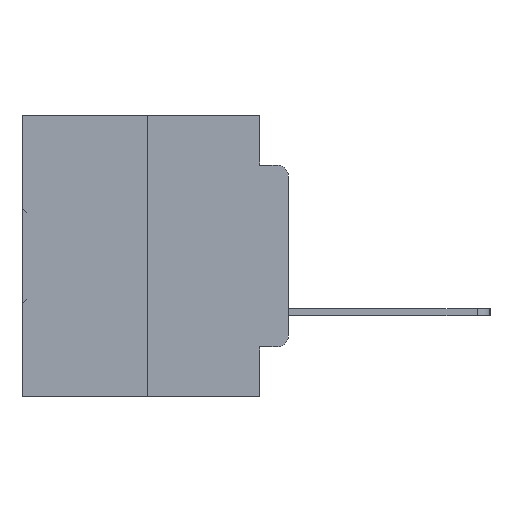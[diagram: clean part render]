
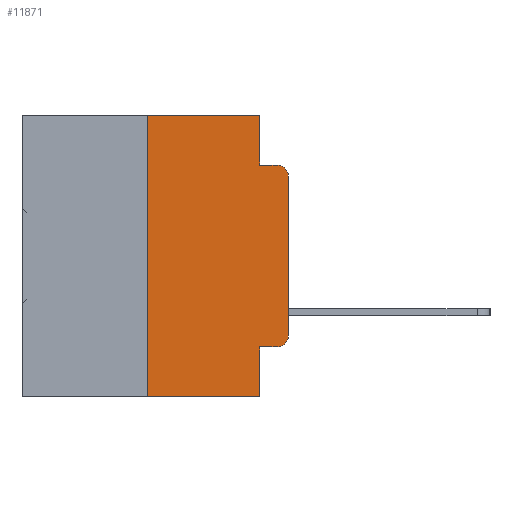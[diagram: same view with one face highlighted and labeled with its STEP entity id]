
A CAD part, left-side view. The second image highlights one B-rep face of the part: STEP entity #11871.
In plain terms, the highlighted planar face has unit normal (-1, 0, 0).
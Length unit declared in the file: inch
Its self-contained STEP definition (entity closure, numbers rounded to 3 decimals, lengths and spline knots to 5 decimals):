
#199 = DIRECTION ( 'NONE',  ( 0., 0., 1. ) ) ;
#475 = VERTEX_POINT ( 'NONE', #21425 ) ;
#478 = EDGE_CURVE ( 'NONE', #475, #26429, #2894, .T. ) ;
#1333 = LINE ( 'NONE', #27882, #20837 ) ;
#1368 = VERTEX_POINT ( 'NONE', #2451 ) ;
#2006 = CARTESIAN_POINT ( 'NONE',  ( 0., 0.051, -0.0885 ) ) ;
#2022 = LINE ( 'NONE', #18140, #21495 ) ;
#2107 = EDGE_CURVE ( 'NONE', #475, #4873, #27811, .T. ) ;
#2392 = CARTESIAN_POINT ( 'NONE',  ( 0., 0.051, 0. ) ) ;
#2451 = CARTESIAN_POINT ( 'NONE',  ( 0., 0., -0.3915 ) ) ;
#2533 = DIRECTION ( 'NONE',  ( 0., -1., 0. ) ) ;
#2737 = CARTESIAN_POINT ( 'NONE',  ( 0., 0.02, -0.4115 ) ) ;
#2894 = LINE ( 'NONE', #4148, #10009 ) ;
#4148 = CARTESIAN_POINT ( 'NONE',  ( 0., 0.25, 0. ) ) ;
#4685 = CARTESIAN_POINT ( 'NONE',  ( 0., 0.25, 0. ) ) ;
#4873 = VERTEX_POINT ( 'NONE', #21176 ) ;
#5117 = CARTESIAN_POINT ( 'NONE',  ( 0., 0., -0.1085 ) ) ;
#5927 = CARTESIAN_POINT ( 'NONE',  ( 0., 0.051, -0.4115 ) ) ;
#6429 = VERTEX_POINT ( 'NONE', #11936 ) ;
#6460 = ORIENTED_EDGE ( 'NONE', *, *, #12528, .T. ) ;
#6681 = VECTOR ( 'NONE', #19303, 39.37008 ) ;
#7149 = EDGE_LOOP ( 'NONE', ( #16428, #6460, #15190, #33262, #27308, #22845, #9764, #24481, #25291, #30917 ) ) ;
#7159 = EDGE_CURVE ( 'NONE', #1368, #19403, #1333, .T. ) ;
#8098 = CIRCLE ( 'NONE', #9084, 0.02 ) ;
#8668 = DIRECTION ( 'NONE',  ( 0., -1., 0. ) ) ;
#8931 = CARTESIAN_POINT ( 'NONE',  ( 0., 0.473, 0. ) ) ;
#9084 = AXIS2_PLACEMENT_3D ( 'NONE', #27501, #11947, #30055 ) ;
#9201 = CIRCLE ( 'NONE', #13900, 0.02 ) ;
#9411 = FACE_OUTER_BOUND ( 'NONE', #7149, .T. ) ;
#9418 = VERTEX_POINT ( 'NONE', #5927 ) ;
#9764 = ORIENTED_EDGE ( 'NONE', *, *, #2107, .T. ) ;
#10009 = VECTOR ( 'NONE', #199, 39.37008 ) ;
#10097 = DIRECTION ( 'NONE',  ( 0., -1., 0. ) ) ;
#11410 = VECTOR ( 'NONE', #10097, 39.37008 ) ;
#11652 = DIRECTION ( 'NONE',  ( 0., 0., -1. ) ) ;
#11871 = ADVANCED_FACE ( 'NONE', ( #9411 ), #22041, .F. ) ;
#11936 = CARTESIAN_POINT ( 'NONE',  ( 0., 0.02, -0.0885 ) ) ;
#11947 = DIRECTION ( 'NONE',  ( -1., 0., 0. ) ) ;
#12125 = VERTEX_POINT ( 'NONE', #2006 ) ;
#12528 = EDGE_CURVE ( 'NONE', #19403, #6429, #8098, .T. ) ;
#13048 = DIRECTION ( 'NONE',  ( -1., 0., 0. ) ) ;
#13287 = CARTESIAN_POINT ( 'NONE',  ( 0., 0.473, 0. ) ) ;
#13429 = VECTOR ( 'NONE', #15507, 39.37008 ) ;
#13900 = AXIS2_PLACEMENT_3D ( 'NONE', #28579, #13048, #31134 ) ;
#14595 = LINE ( 'NONE', #29524, #6681 ) ;
#15190 = ORIENTED_EDGE ( 'NONE', *, *, #32661, .F. ) ;
#15312 = CARTESIAN_POINT ( 'NONE',  ( 0., 0.051, -0.0885 ) ) ;
#15507 = DIRECTION ( 'NONE',  ( 0., 0., -1. ) ) ;
#15632 = DIRECTION ( 'NONE',  ( 0., 0., -1. ) ) ;
#16428 = ORIENTED_EDGE ( 'NONE', *, *, #7159, .T. ) ;
#17356 = VECTOR ( 'NONE', #2533, 39.37008 ) ;
#17895 = EDGE_CURVE ( 'NONE', #9418, #4873, #33975, .T. ) ;
#18140 = CARTESIAN_POINT ( 'NONE',  ( 0., 0.051, 0. ) ) ;
#18176 = LINE ( 'NONE', #13287, #17356 ) ;
#19303 = DIRECTION ( 'NONE',  ( 0., -1., 0. ) ) ;
#19403 = VERTEX_POINT ( 'NONE', #5117 ) ;
#19628 = EDGE_CURVE ( 'NONE', #9418, #29641, #14595, .T. ) ;
#19997 = EDGE_CURVE ( 'NONE', #31754, #12125, #2022, .T. ) ;
#20837 = VECTOR ( 'NONE', #30447, 39.37008 ) ;
#20964 = VECTOR ( 'NONE', #8668, 39.37008 ) ;
#21176 = CARTESIAN_POINT ( 'NONE',  ( 0., 0.051, -0.5 ) ) ;
#21425 = CARTESIAN_POINT ( 'NONE',  ( 0., 0.25, -0.5 ) ) ;
#21495 = VECTOR ( 'NONE', #15632, 39.37008 ) ;
#21791 = CARTESIAN_POINT ( 'NONE',  ( 0., 0.473, -0.5 ) ) ;
#22041 = PLANE ( 'NONE',  #26826 ) ;
#22845 = ORIENTED_EDGE ( 'NONE', *, *, #478, .F. ) ;
#24481 = ORIENTED_EDGE ( 'NONE', *, *, #17895, .F. ) ;
#25291 = ORIENTED_EDGE ( 'NONE', *, *, #19628, .T. ) ;
#26429 = VERTEX_POINT ( 'NONE', #4685 ) ;
#26826 = AXIS2_PLACEMENT_3D ( 'NONE', #8931, #27217, #11652 ) ;
#27192 = EDGE_CURVE ( 'NONE', #29641, #1368, #9201, .T. ) ;
#27217 = DIRECTION ( 'NONE',  ( 1., 0., 0. ) ) ;
#27308 = ORIENTED_EDGE ( 'NONE', *, *, #29011, .F. ) ;
#27501 = CARTESIAN_POINT ( 'NONE',  ( 0., 0.02, -0.1085 ) ) ;
#27811 = LINE ( 'NONE', #21791, #20964 ) ;
#27882 = CARTESIAN_POINT ( 'NONE',  ( 0., 0., 0. ) ) ;
#28579 = CARTESIAN_POINT ( 'NONE',  ( 0., 0.02, -0.3915 ) ) ;
#29011 = EDGE_CURVE ( 'NONE', #26429, #31754, #18176, .T. ) ;
#29524 = CARTESIAN_POINT ( 'NONE',  ( 0., 0.051, -0.4115 ) ) ;
#29641 = VERTEX_POINT ( 'NONE', #2737 ) ;
#30055 = DIRECTION ( 'NONE',  ( 0., 0., -1. ) ) ;
#30447 = DIRECTION ( 'NONE',  ( 0., 0., 1. ) ) ;
#30917 = ORIENTED_EDGE ( 'NONE', *, *, #27192, .T. ) ;
#31134 = DIRECTION ( 'NONE',  ( 0., 0., -1. ) ) ;
#31754 = VERTEX_POINT ( 'NONE', #2392 ) ;
#32661 = EDGE_CURVE ( 'NONE', #12125, #6429, #32827, .T. ) ;
#32827 = LINE ( 'NONE', #15312, #11410 ) ;
#33262 = ORIENTED_EDGE ( 'NONE', *, *, #19997, .F. ) ;
#33493 = CARTESIAN_POINT ( 'NONE',  ( 0., 0.051, 0. ) ) ;
#33975 = LINE ( 'NONE', #33493, #13429 ) ;
